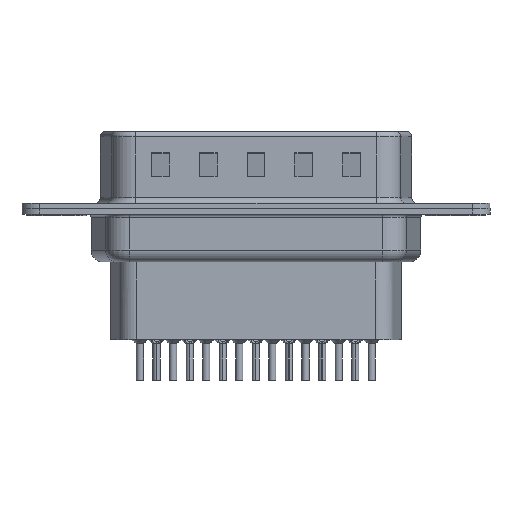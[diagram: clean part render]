
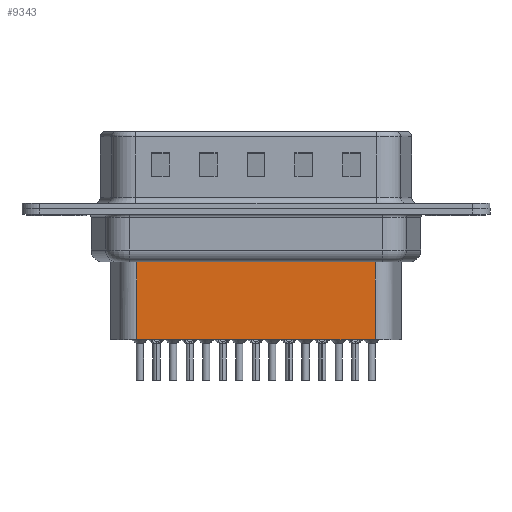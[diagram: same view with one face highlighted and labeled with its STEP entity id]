
A CAD part, front view. The second image highlights one B-rep face of the part: STEP entity #9343.
In plain terms, the highlighted planar face has unit normal (0, -1, 0).
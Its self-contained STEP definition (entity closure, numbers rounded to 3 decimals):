
#144 = AXIS2_PLACEMENT_3D ( 'NONE', #12892, #2426, #11795 ) ;
#310 = LINE ( 'NONE', #9403, #15573 ) ;
#373 = DIRECTION ( 'NONE',  ( 0., 0., -1. ) ) ;
#1104 = CARTESIAN_POINT ( 'NONE',  ( 6.681, -3.5, -10.95 ) ) ;
#1190 = CARTESIAN_POINT ( 'NONE',  ( 6.681, -3.5, -3.1 ) ) ;
#1777 = VERTEX_POINT ( 'NONE', #1104 ) ;
#1796 = EDGE_CURVE ( 'NONE', #2960, #8916, #14741, .T. ) ;
#2245 = ORIENTED_EDGE ( 'NONE', *, *, #1796, .T. ) ;
#2426 = DIRECTION ( 'NONE',  ( 0., -1., 0. ) ) ;
#2960 = VERTEX_POINT ( 'NONE', #9374 ) ;
#3828 = VECTOR ( 'NONE', #19290, 1000. ) ;
#4613 = CARTESIAN_POINT ( 'NONE',  ( 26.619, -3.5, -3.1 ) ) ;
#5879 = CARTESIAN_POINT ( 'NONE',  ( 6.681, -3.5, -4.097 ) ) ;
#5886 = EDGE_CURVE ( 'NONE', #2960, #6636, #12325, .T. ) ;
#6636 = VERTEX_POINT ( 'NONE', #15524 ) ;
#7075 = EDGE_CURVE ( 'NONE', #6636, #1777, #310, .T. ) ;
#8526 = ORIENTED_EDGE ( 'NONE', *, *, #7075, .F. ) ;
#8916 = VERTEX_POINT ( 'NONE', #5879 ) ;
#9343 = ADVANCED_FACE ( 'NONE', ( #11705 ), #17510, .T. ) ;
#9374 = CARTESIAN_POINT ( 'NONE',  ( 26.619, -3.5, -4.097 ) ) ;
#9403 = CARTESIAN_POINT ( 'NONE',  ( 6.681, -3.5, -10.95 ) ) ;
#11705 = FACE_OUTER_BOUND ( 'NONE', #14522, .T. ) ;
#11795 = DIRECTION ( 'NONE',  ( 1., 0., 0. ) ) ;
#12325 = LINE ( 'NONE', #4613, #16165 ) ;
#12351 = DIRECTION ( 'NONE',  ( -1., 0., 0. ) ) ;
#12502 = ORIENTED_EDGE ( 'NONE', *, *, #13715, .T. ) ;
#12874 = VECTOR ( 'NONE', #14827, 1000. ) ;
#12892 = CARTESIAN_POINT ( 'NONE',  ( 6.681, -3.5, -3.1 ) ) ;
#13062 = CARTESIAN_POINT ( 'NONE',  ( 6.434, -3.5, -4.097 ) ) ;
#13715 = EDGE_CURVE ( 'NONE', #8916, #1777, #14917, .T. ) ;
#14522 = EDGE_LOOP ( 'NONE', ( #17844, #2245, #12502, #8526 ) ) ;
#14741 = LINE ( 'NONE', #13062, #3828 ) ;
#14827 = DIRECTION ( 'NONE',  ( 0., 0., -1. ) ) ;
#14917 = LINE ( 'NONE', #1190, #12874 ) ;
#15524 = CARTESIAN_POINT ( 'NONE',  ( 26.619, -3.5, -10.95 ) ) ;
#15573 = VECTOR ( 'NONE', #12351, 1000. ) ;
#16165 = VECTOR ( 'NONE', #373, 1000. ) ;
#17510 = PLANE ( 'NONE',  #144 ) ;
#17844 = ORIENTED_EDGE ( 'NONE', *, *, #5886, .F. ) ;
#19290 = DIRECTION ( 'NONE',  ( -1., 0., 0. ) ) ;
